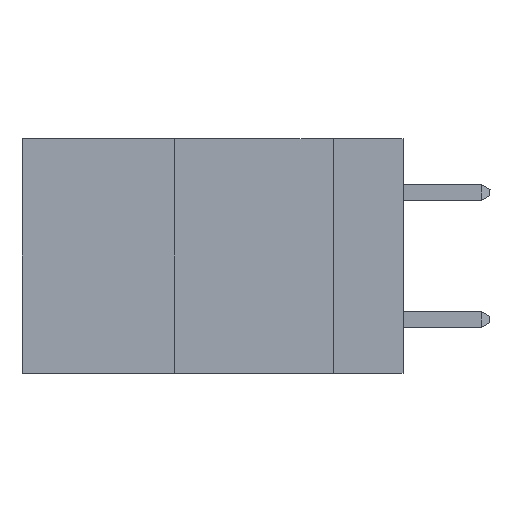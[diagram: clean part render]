
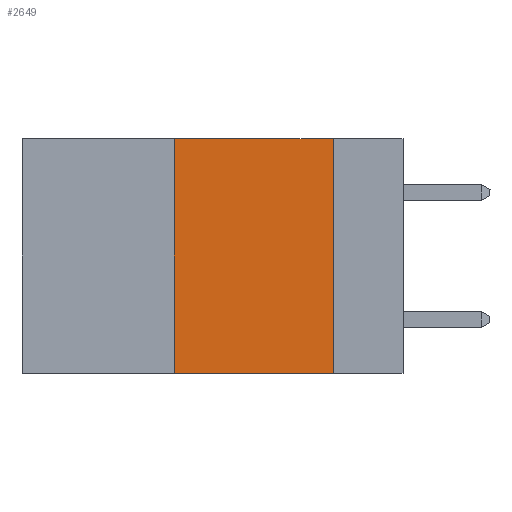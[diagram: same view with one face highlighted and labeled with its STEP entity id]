
A CAD part, left-side view. The second image highlights one B-rep face of the part: STEP entity #2649.
In plain terms, the highlighted planar face has unit normal (-1, 0, 0).
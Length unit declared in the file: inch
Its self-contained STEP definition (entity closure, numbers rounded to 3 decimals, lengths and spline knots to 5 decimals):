
#410 = ORIENTED_EDGE ( 'NONE', *, *, #5197, .F. ) ;
#944 = EDGE_CURVE ( 'NONE', #8559, #9664, #10475, .T. ) ;
#1161 = LINE ( 'NONE', #9637, #2741 ) ;
#1237 = CARTESIAN_POINT ( 'NONE',  ( 0., 0.6, 0. ) ) ;
#1413 = VECTOR ( 'NONE', #9370, 39.37008 ) ;
#1460 = PLANE ( 'NONE',  #3432 ) ;
#2360 = DIRECTION ( 'NONE',  ( 0., -1., 0. ) ) ;
#2487 = VERTEX_POINT ( 'NONE', #2958 ) ;
#2627 = VERTEX_POINT ( 'NONE', #6607 ) ;
#2649 = ADVANCED_FACE ( 'NONE', ( #3874 ), #1460, .F. ) ;
#2741 = VECTOR ( 'NONE', #5375, 39.37008 ) ;
#2891 = DIRECTION ( 'NONE',  ( 0., -1., 0. ) ) ;
#2958 = CARTESIAN_POINT ( 'NONE',  ( 0., 0.36, 0. ) ) ;
#2964 = EDGE_CURVE ( 'NONE', #2487, #8559, #8857, .T. ) ;
#3432 = AXIS2_PLACEMENT_3D ( 'NONE', #10829, #4946, #7429 ) ;
#3874 = FACE_OUTER_BOUND ( 'NONE', #6038, .T. ) ;
#4946 = DIRECTION ( 'NONE',  ( 1., 0., 0. ) ) ;
#5124 = ORIENTED_EDGE ( 'NONE', *, *, #944, .F. ) ;
#5197 = EDGE_CURVE ( 'NONE', #2627, #2487, #1161, .T. ) ;
#5375 = DIRECTION ( 'NONE',  ( 0., 0., 1. ) ) ;
#5629 = LINE ( 'NONE', #5710, #7541 ) ;
#5710 = CARTESIAN_POINT ( 'NONE',  ( 0., 0.6, -0.37 ) ) ;
#5889 = EDGE_CURVE ( 'NONE', #2627, #9664, #5629, .T. ) ;
#6038 = EDGE_LOOP ( 'NONE', ( #5124, #9799, #410, #9727 ) ) ;
#6607 = CARTESIAN_POINT ( 'NONE',  ( 0., 0.36, -0.37 ) ) ;
#7429 = DIRECTION ( 'NONE',  ( 0., 0., -1. ) ) ;
#7541 = VECTOR ( 'NONE', #2360, 39.37008 ) ;
#8372 = CARTESIAN_POINT ( 'NONE',  ( 0., 0.11, 0. ) ) ;
#8559 = VERTEX_POINT ( 'NONE', #8372 ) ;
#8857 = LINE ( 'NONE', #1237, #9006 ) ;
#8891 = CARTESIAN_POINT ( 'NONE',  ( 0., 0.11, -0.37 ) ) ;
#9006 = VECTOR ( 'NONE', #2891, 39.37008 ) ;
#9370 = DIRECTION ( 'NONE',  ( 0., 0., -1. ) ) ;
#9637 = CARTESIAN_POINT ( 'NONE',  ( 0., 0.36, 0. ) ) ;
#9664 = VERTEX_POINT ( 'NONE', #8891 ) ;
#9727 = ORIENTED_EDGE ( 'NONE', *, *, #5889, .T. ) ;
#9799 = ORIENTED_EDGE ( 'NONE', *, *, #2964, .F. ) ;
#10144 = CARTESIAN_POINT ( 'NONE',  ( 0., 0.11, 0. ) ) ;
#10475 = LINE ( 'NONE', #10144, #1413 ) ;
#10829 = CARTESIAN_POINT ( 'NONE',  ( 0., 0.6, 0. ) ) ;
